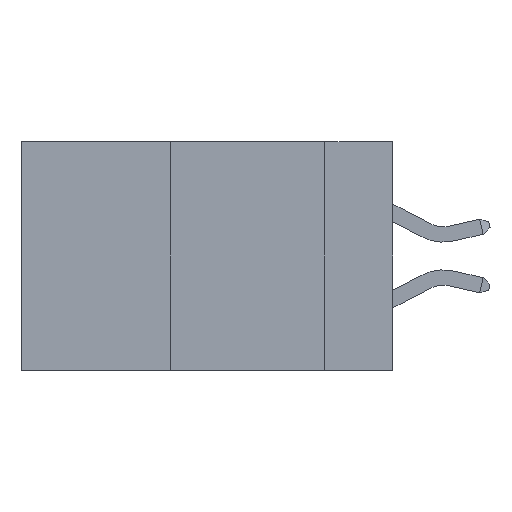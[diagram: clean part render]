
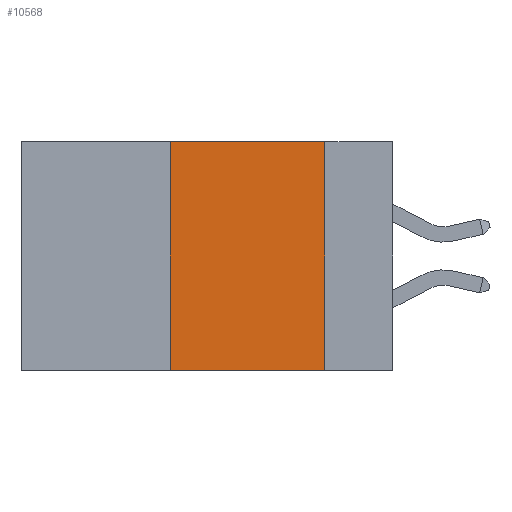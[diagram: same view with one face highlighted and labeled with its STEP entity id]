
A CAD part, left-side view. The second image highlights one B-rep face of the part: STEP entity #10568.
In plain terms, the highlighted planar face has unit normal (-1, 0, 0).
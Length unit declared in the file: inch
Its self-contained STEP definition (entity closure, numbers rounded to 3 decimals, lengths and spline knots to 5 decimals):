
#70 = EDGE_LOOP ( 'NONE', ( #14885, #2312, #4711, #1276 ) ) ;
#359 = VERTEX_POINT ( 'NONE', #6510 ) ;
#371 = CARTESIAN_POINT ( 'NONE',  ( 0., 0.6, 0. ) ) ;
#388 = DIRECTION ( 'NONE',  ( 0., -1., 0. ) ) ;
#1276 = ORIENTED_EDGE ( 'NONE', *, *, #11285, .T. ) ;
#1321 = VECTOR ( 'NONE', #11561, 39.37008 ) ;
#1990 = LINE ( 'NONE', #12765, #10892 ) ;
#2312 = ORIENTED_EDGE ( 'NONE', *, *, #4003, .F. ) ;
#2516 = PLANE ( 'NONE',  #5663 ) ;
#3012 = FACE_OUTER_BOUND ( 'NONE', #70, .T. ) ;
#3688 = DIRECTION ( 'NONE',  ( 0., 0., -1. ) ) ;
#4003 = EDGE_CURVE ( 'NONE', #359, #12280, #6466, .T. ) ;
#4354 = EDGE_CURVE ( 'NONE', #12280, #11834, #1990, .T. ) ;
#4502 = LINE ( 'NONE', #8161, #1321 ) ;
#4569 = VERTEX_POINT ( 'NONE', #7438 ) ;
#4711 = ORIENTED_EDGE ( 'NONE', *, *, #10431, .F. ) ;
#5663 = AXIS2_PLACEMENT_3D ( 'NONE', #12854, #10615, #3688 ) ;
#6466 = LINE ( 'NONE', #371, #9501 ) ;
#6510 = CARTESIAN_POINT ( 'NONE',  ( 0., 0.36, 0. ) ) ;
#7438 = CARTESIAN_POINT ( 'NONE',  ( 0., 0.36, -0.37 ) ) ;
#7959 = VECTOR ( 'NONE', #13028, 39.37008 ) ;
#8161 = CARTESIAN_POINT ( 'NONE',  ( 0., 0.36, 0. ) ) ;
#9501 = VECTOR ( 'NONE', #388, 39.37008 ) ;
#10431 = EDGE_CURVE ( 'NONE', #4569, #359, #4502, .T. ) ;
#10437 = CARTESIAN_POINT ( 'NONE',  ( 0., 0.11, -0.37 ) ) ;
#10568 = ADVANCED_FACE ( 'NONE', ( #3012 ), #2516, .F. ) ;
#10615 = DIRECTION ( 'NONE',  ( 1., 0., 0. ) ) ;
#10892 = VECTOR ( 'NONE', #13939, 39.37008 ) ;
#11285 = EDGE_CURVE ( 'NONE', #4569, #11834, #14022, .T. ) ;
#11561 = DIRECTION ( 'NONE',  ( 0., 0., 1. ) ) ;
#11834 = VERTEX_POINT ( 'NONE', #10437 ) ;
#11888 = CARTESIAN_POINT ( 'NONE',  ( 0., 0.6, -0.37 ) ) ;
#12280 = VERTEX_POINT ( 'NONE', #13825 ) ;
#12765 = CARTESIAN_POINT ( 'NONE',  ( 0., 0.11, 0. ) ) ;
#12854 = CARTESIAN_POINT ( 'NONE',  ( 0., 0.6, 0. ) ) ;
#13028 = DIRECTION ( 'NONE',  ( 0., -1., 0. ) ) ;
#13825 = CARTESIAN_POINT ( 'NONE',  ( 0., 0.11, 0. ) ) ;
#13939 = DIRECTION ( 'NONE',  ( 0., 0., -1. ) ) ;
#14022 = LINE ( 'NONE', #11888, #7959 ) ;
#14885 = ORIENTED_EDGE ( 'NONE', *, *, #4354, .F. ) ;
